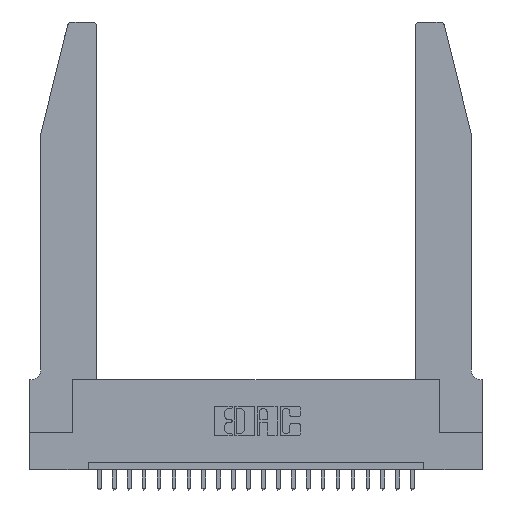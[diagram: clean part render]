
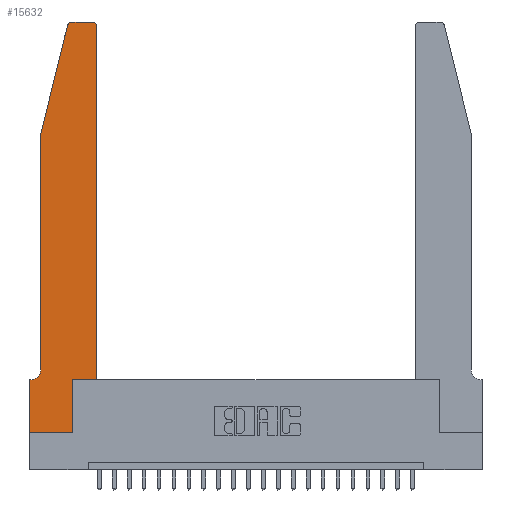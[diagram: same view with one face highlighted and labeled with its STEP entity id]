
A CAD part, top view. The second image highlights one B-rep face of the part: STEP entity #15632.
In plain terms, the highlighted planar face has unit normal (0, 0, 1).
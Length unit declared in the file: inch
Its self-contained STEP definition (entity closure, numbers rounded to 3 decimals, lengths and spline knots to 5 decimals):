
#138 = CARTESIAN_POINT ( 'NONE',  ( 0., 0.35, 0.37 ) ) ;
#460 = DIRECTION ( 'NONE',  ( 0., 0., 1. ) ) ;
#706 = CARTESIAN_POINT ( 'NONE',  ( 0.2865, 0., 0.37 ) ) ;
#802 = ORIENTED_EDGE ( 'NONE', *, *, #3980, .T. ) ;
#856 = LINE ( 'NONE', #11078, #20270 ) ;
#1028 = CARTESIAN_POINT ( 'NONE',  ( 0.25487, 2.72718, 0.37 ) ) ;
#1193 = LINE ( 'NONE', #18096, #16534 ) ;
#1294 = ORIENTED_EDGE ( 'NONE', *, *, #9361, .T. ) ;
#1474 = VERTEX_POINT ( 'NONE', #19190 ) ;
#1547 = ORIENTED_EDGE ( 'NONE', *, *, #12997, .T. ) ;
#1687 = ORIENTED_EDGE ( 'NONE', *, *, #5037, .T. ) ;
#1942 = ORIENTED_EDGE ( 'NONE', *, *, #9204, .T. ) ;
#2637 = FACE_OUTER_BOUND ( 'NONE', #23591, .T. ) ;
#2763 = CARTESIAN_POINT ( 'NONE',  ( 0.4505, 0.35, 0.37 ) ) ;
#3129 = VERTEX_POINT ( 'NONE', #9737 ) ;
#3163 = EDGE_CURVE ( 'NONE', #8990, #14720, #9167, .T. ) ;
#3247 = DIRECTION ( 'NONE',  ( 0., 1., 0. ) ) ;
#3411 = DIRECTION ( 'NONE',  ( -0.239, -0.971, 0. ) ) ;
#3604 = DIRECTION ( 'NONE',  ( 0., 1., 0. ) ) ;
#3980 = EDGE_CURVE ( 'NONE', #18472, #6426, #22734, .T. ) ;
#3985 = CARTESIAN_POINT ( 'NONE',  ( 0.2605, 2.75, 0.37 ) ) ;
#4577 = EDGE_CURVE ( 'NONE', #12732, #3129, #7710, .T. ) ;
#4676 = ORIENTED_EDGE ( 'NONE', *, *, #14192, .T. ) ;
#4879 = CARTESIAN_POINT ( 'NONE',  ( 0.0055, 0.35, 0.37 ) ) ;
#4935 = EDGE_CURVE ( 'NONE', #15605, #7815, #7408, .T. ) ;
#5037 = EDGE_CURVE ( 'NONE', #5778, #12732, #21289, .T. ) ;
#5200 = LINE ( 'NONE', #7415, #8670 ) ;
#5753 = ORIENTED_EDGE ( 'NONE', *, *, #3163, .T. ) ;
#5778 = VERTEX_POINT ( 'NONE', #8170 ) ;
#6048 = CARTESIAN_POINT ( 'NONE',  ( 0.4205, 2.72, 0.37 ) ) ;
#6120 = AXIS2_PLACEMENT_3D ( 'NONE', #14094, #6775, #12681 ) ;
#6313 = DIRECTION ( 'NONE',  ( 1., 0., 0. ) ) ;
#6426 = VERTEX_POINT ( 'NONE', #4879 ) ;
#6775 = DIRECTION ( 'NONE',  ( 0., 0., 1. ) ) ;
#7283 = EDGE_CURVE ( 'NONE', #20498, #8990, #856, .T. ) ;
#7380 = DIRECTION ( 'NONE',  ( 0., -1., 0. ) ) ;
#7408 = LINE ( 'NONE', #12902, #17503 ) ;
#7415 = CARTESIAN_POINT ( 'NONE',  ( 0.0755, 2., 0.37 ) ) ;
#7710 = LINE ( 'NONE', #3985, #9668 ) ;
#7815 = VERTEX_POINT ( 'NONE', #17339 ) ;
#8114 = CARTESIAN_POINT ( 'NONE',  ( 0.0055, 0.42, 0.37 ) ) ;
#8170 = CARTESIAN_POINT ( 'NONE',  ( 0.4505, 2.72, 0.37 ) ) ;
#8315 = AXIS2_PLACEMENT_3D ( 'NONE', #8114, #12263, #9929 ) ;
#8670 = VECTOR ( 'NONE', #20352, 39.37008 ) ;
#8990 = VERTEX_POINT ( 'NONE', #16038 ) ;
#9167 = LINE ( 'NONE', #9988, #19618 ) ;
#9204 = EDGE_CURVE ( 'NONE', #14720, #5778, #23486, .T. ) ;
#9361 = EDGE_CURVE ( 'NONE', #6426, #15605, #14491, .T. ) ;
#9668 = VECTOR ( 'NONE', #9734, 39.37008 ) ;
#9734 = DIRECTION ( 'NONE',  ( -1., 0., 0. ) ) ;
#9737 = CARTESIAN_POINT ( 'NONE',  ( 0.284, 2.75, 0.37 ) ) ;
#9929 = DIRECTION ( 'NONE',  ( -1., 0., 0. ) ) ;
#9988 = CARTESIAN_POINT ( 'NONE',  ( 0.4505, 0.35, 0.37 ) ) ;
#11078 = CARTESIAN_POINT ( 'NONE',  ( 0.2865, 0.35, 0.37 ) ) ;
#11146 = VECTOR ( 'NONE', #22937, 39.37008 ) ;
#11598 = CARTESIAN_POINT ( 'NONE',  ( 0.4205, 2.75, 0.37 ) ) ;
#11813 = ORIENTED_EDGE ( 'NONE', *, *, #7283, .T. ) ;
#11856 = DIRECTION ( 'NONE',  ( 1., 0., 0. ) ) ;
#11995 = ORIENTED_EDGE ( 'NONE', *, *, #17192, .T. ) ;
#12161 = ORIENTED_EDGE ( 'NONE', *, *, #15527, .T. ) ;
#12263 = DIRECTION ( 'NONE',  ( 0., 0., -1. ) ) ;
#12681 = DIRECTION ( 'NONE',  ( 1., 0., 0. ) ) ;
#12732 = VERTEX_POINT ( 'NONE', #11598 ) ;
#12737 = VECTOR ( 'NONE', #13223, 39.37008 ) ;
#12902 = CARTESIAN_POINT ( 'NONE',  ( 0., 0., 0.37 ) ) ;
#12997 = EDGE_CURVE ( 'NONE', #7815, #20498, #16344, .T. ) ;
#13223 = DIRECTION ( 'NONE',  ( -1., 0., 0. ) ) ;
#13768 = DIRECTION ( 'NONE',  ( 1., 0., 0. ) ) ;
#13840 = PLANE ( 'NONE',  #6120 ) ;
#14094 = CARTESIAN_POINT ( 'NONE',  ( 0., 0.35, 0.37 ) ) ;
#14192 = EDGE_CURVE ( 'NONE', #3129, #19017, #22392, .T. ) ;
#14491 = LINE ( 'NONE', #16964, #12737 ) ;
#14720 = VERTEX_POINT ( 'NONE', #2763 ) ;
#15527 = EDGE_CURVE ( 'NONE', #19017, #1474, #1193, .T. ) ;
#15605 = VERTEX_POINT ( 'NONE', #138 ) ;
#15632 = ADVANCED_FACE ( 'NONE', ( #2637 ), #13840, .T. ) ;
#16038 = CARTESIAN_POINT ( 'NONE',  ( 0.2865, 0.35, 0.37 ) ) ;
#16344 = LINE ( 'NONE', #17493, #11146 ) ;
#16534 = VECTOR ( 'NONE', #3411, 39.37008 ) ;
#16936 = AXIS2_PLACEMENT_3D ( 'NONE', #23465, #460, #6313 ) ;
#16964 = CARTESIAN_POINT ( 'NONE',  ( 0.0755, 0.35, 0.37 ) ) ;
#17189 = ORIENTED_EDGE ( 'NONE', *, *, #4935, .T. ) ;
#17192 = EDGE_CURVE ( 'NONE', #1474, #18472, #5200, .T. ) ;
#17339 = CARTESIAN_POINT ( 'NONE',  ( 0., 0., 0.37 ) ) ;
#17493 = CARTESIAN_POINT ( 'NONE',  ( 0., 0., 0.37 ) ) ;
#17503 = VECTOR ( 'NONE', #7380, 39.37008 ) ;
#17692 = VECTOR ( 'NONE', #3247, 39.37008 ) ;
#18096 = CARTESIAN_POINT ( 'NONE',  ( 0.0755, 2., 0.37 ) ) ;
#18472 = VERTEX_POINT ( 'NONE', #21233 ) ;
#19017 = VERTEX_POINT ( 'NONE', #1028 ) ;
#19190 = CARTESIAN_POINT ( 'NONE',  ( 0.0755, 2., 0.37 ) ) ;
#19618 = VECTOR ( 'NONE', #13768, 39.37008 ) ;
#19899 = CARTESIAN_POINT ( 'NONE',  ( 0.4505, 0.35, 0.37 ) ) ;
#20270 = VECTOR ( 'NONE', #3604, 39.37008 ) ;
#20352 = DIRECTION ( 'NONE',  ( 0., -1., 0. ) ) ;
#20498 = VERTEX_POINT ( 'NONE', #706 ) ;
#20547 = AXIS2_PLACEMENT_3D ( 'NONE', #6048, #21109, #11856 ) ;
#21109 = DIRECTION ( 'NONE',  ( 0., 0., 1. ) ) ;
#21233 = CARTESIAN_POINT ( 'NONE',  ( 0.0755, 0.42, 0.37 ) ) ;
#21289 = CIRCLE ( 'NONE', #20547, 0.03 ) ;
#22392 = CIRCLE ( 'NONE', #16936, 0.03 ) ;
#22590 = ORIENTED_EDGE ( 'NONE', *, *, #4577, .T. ) ;
#22734 = CIRCLE ( 'NONE', #8315, 0.07 ) ;
#22937 = DIRECTION ( 'NONE',  ( 1., 0., 0. ) ) ;
#23465 = CARTESIAN_POINT ( 'NONE',  ( 0.284, 2.72, 0.37 ) ) ;
#23486 = LINE ( 'NONE', #19899, #17692 ) ;
#23591 = EDGE_LOOP ( 'NONE', ( #22590, #4676, #12161, #11995, #802, #1294, #17189, #1547, #11813, #5753, #1942, #1687 ) ) ;
